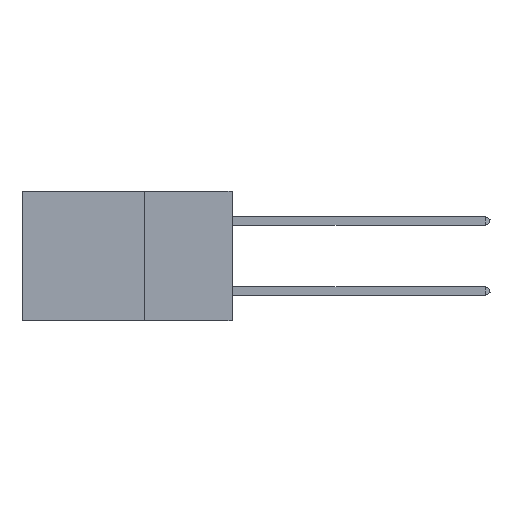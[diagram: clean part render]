
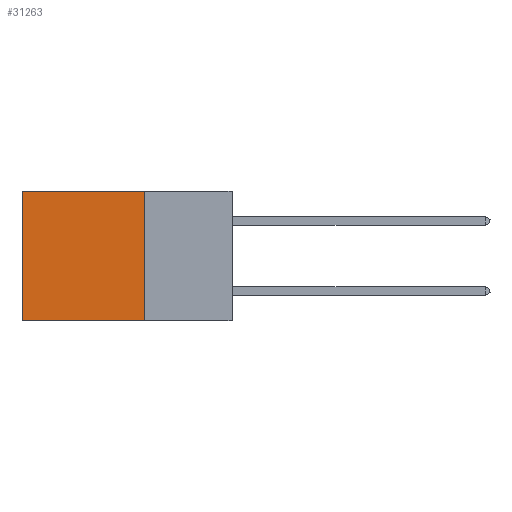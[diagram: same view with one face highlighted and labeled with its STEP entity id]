
A CAD part, left-side view. The second image highlights one B-rep face of the part: STEP entity #31263.
In plain terms, the highlighted planar face has unit normal (-1, 0, 0).
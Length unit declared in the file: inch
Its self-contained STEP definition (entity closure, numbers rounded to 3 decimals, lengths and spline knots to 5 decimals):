
#960 = EDGE_CURVE ( 'NONE', #41667, #42653, #10630, .T. ) ;
#3077 = VECTOR ( 'NONE', #38000, 39.37008 ) ;
#3978 = CARTESIAN_POINT ( 'NONE',  ( 0.2875, 0.25, 0. ) ) ;
#6083 = DIRECTION ( 'NONE',  ( 0., 0., -1. ) ) ;
#8016 = CARTESIAN_POINT ( 'NONE',  ( 0.2875, 0.25, 0. ) ) ;
#10550 = DIRECTION ( 'NONE',  ( 0., 1., 0. ) ) ;
#10630 = LINE ( 'NONE', #29343, #30581 ) ;
#10873 = EDGE_LOOP ( 'NONE', ( #27062, #43702, #42937, #42232 ) ) ;
#12821 = CARTESIAN_POINT ( 'NONE',  ( 0.2875, 0.6, 0. ) ) ;
#13104 = EDGE_CURVE ( 'NONE', #42467, #16427, #20356, .T. ) ;
#13863 = VECTOR ( 'NONE', #10550, 39.37008 ) ;
#14827 = DIRECTION ( 'NONE',  ( 0., 0., -1. ) ) ;
#16427 = VERTEX_POINT ( 'NONE', #12821 ) ;
#19819 = CARTESIAN_POINT ( 'NONE',  ( 0.2875, 0.25, 0. ) ) ;
#20356 = LINE ( 'NONE', #31082, #13863 ) ;
#20584 = CARTESIAN_POINT ( 'NONE',  ( 0.2875, 0.6, 0. ) ) ;
#23309 = DIRECTION ( 'NONE',  ( 1., 0., 0. ) ) ;
#23826 = CARTESIAN_POINT ( 'NONE',  ( 0.2875, 0.25, -0.37 ) ) ;
#27062 = ORIENTED_EDGE ( 'NONE', *, *, #38563, .T. ) ;
#28451 = EDGE_CURVE ( 'NONE', #42467, #41667, #39629, .T. ) ;
#29343 = CARTESIAN_POINT ( 'NONE',  ( 0.2875, 0.25, -0.37 ) ) ;
#30581 = VECTOR ( 'NONE', #36232, 39.37008 ) ;
#30859 = CARTESIAN_POINT ( 'NONE',  ( 0.2875, 0.6, -0.37 ) ) ;
#31082 = CARTESIAN_POINT ( 'NONE',  ( 0.2875, 0.25, 0. ) ) ;
#31263 = ADVANCED_FACE ( 'NONE', ( #31820 ), #40442, .F. ) ;
#31820 = FACE_OUTER_BOUND ( 'NONE', #10873, .T. ) ;
#32077 = VECTOR ( 'NONE', #14827, 39.37008 ) ;
#34689 = AXIS2_PLACEMENT_3D ( 'NONE', #19819, #23309, #6083 ) ;
#36232 = DIRECTION ( 'NONE',  ( 0., 1., 0. ) ) ;
#38000 = DIRECTION ( 'NONE',  ( 0., 0., -1. ) ) ;
#38563 = EDGE_CURVE ( 'NONE', #16427, #42653, #40802, .T. ) ;
#39629 = LINE ( 'NONE', #8016, #32077 ) ;
#40442 = PLANE ( 'NONE',  #34689 ) ;
#40802 = LINE ( 'NONE', #20584, #3077 ) ;
#41667 = VERTEX_POINT ( 'NONE', #23826 ) ;
#42232 = ORIENTED_EDGE ( 'NONE', *, *, #13104, .T. ) ;
#42467 = VERTEX_POINT ( 'NONE', #3978 ) ;
#42653 = VERTEX_POINT ( 'NONE', #30859 ) ;
#42937 = ORIENTED_EDGE ( 'NONE', *, *, #28451, .F. ) ;
#43702 = ORIENTED_EDGE ( 'NONE', *, *, #960, .F. ) ;
